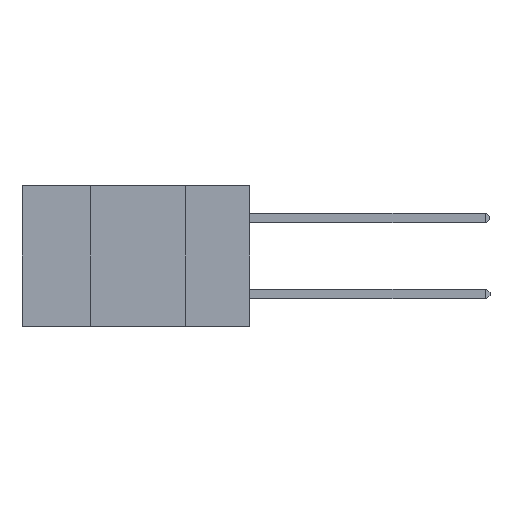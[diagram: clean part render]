
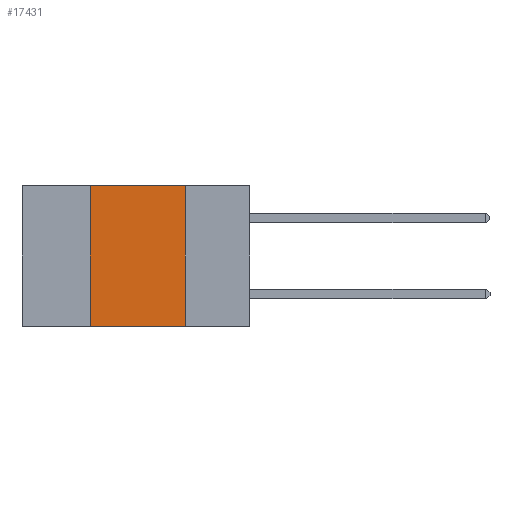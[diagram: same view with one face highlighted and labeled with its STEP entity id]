
A CAD part, left-side view. The second image highlights one B-rep face of the part: STEP entity #17431.
In plain terms, the highlighted planar face has unit normal (-1, 0, 0).
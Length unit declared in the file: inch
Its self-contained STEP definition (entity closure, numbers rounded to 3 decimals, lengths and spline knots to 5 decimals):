
#375 = CARTESIAN_POINT ( 'NONE',  ( 0., 0.42, -0.37 ) ) ;
#1081 = FACE_OUTER_BOUND ( 'NONE', #9923, .T. ) ;
#1751 = ORIENTED_EDGE ( 'NONE', *, *, #7464, .F. ) ;
#2722 = DIRECTION ( 'NONE',  ( 0., -1., 0. ) ) ;
#2997 = LINE ( 'NONE', #18537, #14860 ) ;
#3300 = VECTOR ( 'NONE', #2722, 39.37008 ) ;
#3470 = PLANE ( 'NONE',  #5749 ) ;
#3619 = VECTOR ( 'NONE', #10720, 39.37008 ) ;
#4614 = CARTESIAN_POINT ( 'NONE',  ( 0., 0.6, -0.37 ) ) ;
#4660 = CARTESIAN_POINT ( 'NONE',  ( 0., 0.42, 0. ) ) ;
#5090 = DIRECTION ( 'NONE',  ( 0., 0., -1. ) ) ;
#5749 = AXIS2_PLACEMENT_3D ( 'NONE', #19384, #14715, #5090 ) ;
#7057 = ORIENTED_EDGE ( 'NONE', *, *, #19068, .F. ) ;
#7464 = EDGE_CURVE ( 'NONE', #19112, #11443, #16119, .T. ) ;
#8401 = EDGE_CURVE ( 'NONE', #20100, #13564, #10822, .T. ) ;
#8977 = DIRECTION ( 'NONE',  ( 0., 0., -1. ) ) ;
#9097 = CARTESIAN_POINT ( 'NONE',  ( 0., 0.42, 0. ) ) ;
#9695 = ORIENTED_EDGE ( 'NONE', *, *, #14881, .F. ) ;
#9923 = EDGE_LOOP ( 'NONE', ( #9695, #1751, #7057, #19046 ) ) ;
#10031 = CARTESIAN_POINT ( 'NONE',  ( 0., 0.17, 0. ) ) ;
#10308 = VECTOR ( 'NONE', #15921, 39.37008 ) ;
#10720 = DIRECTION ( 'NONE',  ( 0., 0., 1. ) ) ;
#10822 = LINE ( 'NONE', #4614, #10308 ) ;
#11443 = VERTEX_POINT ( 'NONE', #10031 ) ;
#13564 = VERTEX_POINT ( 'NONE', #16934 ) ;
#14715 = DIRECTION ( 'NONE',  ( 1., 0., 0. ) ) ;
#14860 = VECTOR ( 'NONE', #8977, 39.37008 ) ;
#14881 = EDGE_CURVE ( 'NONE', #11443, #13564, #2997, .T. ) ;
#15546 = CARTESIAN_POINT ( 'NONE',  ( 0., 0.6, 0. ) ) ;
#15921 = DIRECTION ( 'NONE',  ( 0., -1., 0. ) ) ;
#16119 = LINE ( 'NONE', #15546, #3300 ) ;
#16906 = LINE ( 'NONE', #9097, #3619 ) ;
#16934 = CARTESIAN_POINT ( 'NONE',  ( 0., 0.17, -0.37 ) ) ;
#17431 = ADVANCED_FACE ( 'NONE', ( #1081 ), #3470, .F. ) ;
#18537 = CARTESIAN_POINT ( 'NONE',  ( 0., 0.17, 0. ) ) ;
#19046 = ORIENTED_EDGE ( 'NONE', *, *, #8401, .T. ) ;
#19068 = EDGE_CURVE ( 'NONE', #20100, #19112, #16906, .T. ) ;
#19112 = VERTEX_POINT ( 'NONE', #4660 ) ;
#19384 = CARTESIAN_POINT ( 'NONE',  ( 0., 0.6, 0. ) ) ;
#20100 = VERTEX_POINT ( 'NONE', #375 ) ;
